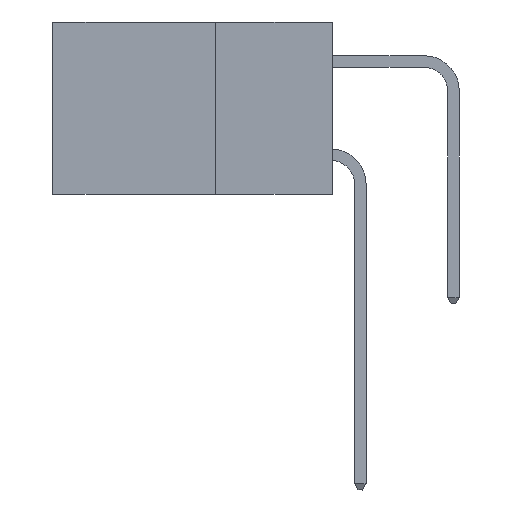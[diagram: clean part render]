
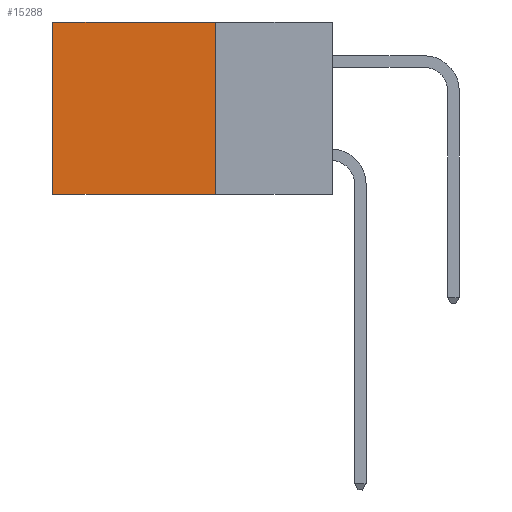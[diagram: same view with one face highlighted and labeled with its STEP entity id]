
A CAD part, left-side view. The second image highlights one B-rep face of the part: STEP entity #15288.
In plain terms, the highlighted planar face has unit normal (-1, 0, 0).
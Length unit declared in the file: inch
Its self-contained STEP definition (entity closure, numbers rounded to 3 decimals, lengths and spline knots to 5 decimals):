
#237 = CARTESIAN_POINT ( 'NONE',  ( 0.2615, 0.6, -0.37 ) ) ;
#735 = VERTEX_POINT ( 'NONE', #8768 ) ;
#882 = EDGE_CURVE ( 'NONE', #735, #15357, #3369, .T. ) ;
#1232 = VECTOR ( 'NONE', #13701, 39.37008 ) ;
#1539 = CARTESIAN_POINT ( 'NONE',  ( 0.2615, 0.6, 0. ) ) ;
#2678 = LINE ( 'NONE', #19272, #17702 ) ;
#2715 = ORIENTED_EDGE ( 'NONE', *, *, #5434, .F. ) ;
#2797 = DIRECTION ( 'NONE',  ( 0., 0., -1. ) ) ;
#2817 = LINE ( 'NONE', #7507, #16532 ) ;
#3369 = LINE ( 'NONE', #16839, #11816 ) ;
#3774 = EDGE_CURVE ( 'NONE', #735, #16047, #2678, .T. ) ;
#3969 = ORIENTED_EDGE ( 'NONE', *, *, #882, .F. ) ;
#4249 = CARTESIAN_POINT ( 'NONE',  ( 0.2615, 0.25, -0.37 ) ) ;
#5434 = EDGE_CURVE ( 'NONE', #15357, #15599, #2817, .T. ) ;
#5747 = CARTESIAN_POINT ( 'NONE',  ( 0.2615, 0.25, -0.37 ) ) ;
#6977 = DIRECTION ( 'NONE',  ( 0., 1., 0. ) ) ;
#7190 = ORIENTED_EDGE ( 'NONE', *, *, #8934, .T. ) ;
#7507 = CARTESIAN_POINT ( 'NONE',  ( 0.2615, 0.25, -0.37 ) ) ;
#8630 = DIRECTION ( 'NONE',  ( 0., 0., -1. ) ) ;
#8768 = CARTESIAN_POINT ( 'NONE',  ( 0.2615, 0.25, 0. ) ) ;
#8934 = EDGE_CURVE ( 'NONE', #16047, #15599, #16800, .T. ) ;
#9025 = PLANE ( 'NONE',  #16343 ) ;
#11723 = DIRECTION ( 'NONE',  ( 1., 0., 0. ) ) ;
#11816 = VECTOR ( 'NONE', #2797, 39.37008 ) ;
#12536 = CARTESIAN_POINT ( 'NONE',  ( 0.2615, 0.6, -0.37 ) ) ;
#13701 = DIRECTION ( 'NONE',  ( 0., 0., -1. ) ) ;
#15288 = ADVANCED_FACE ( 'NONE', ( #16522 ), #9025, .F. ) ;
#15357 = VERTEX_POINT ( 'NONE', #4249 ) ;
#15599 = VERTEX_POINT ( 'NONE', #12536 ) ;
#16047 = VERTEX_POINT ( 'NONE', #1539 ) ;
#16343 = AXIS2_PLACEMENT_3D ( 'NONE', #5747, #11723, #8630 ) ;
#16389 = DIRECTION ( 'NONE',  ( 0., 1., 0. ) ) ;
#16522 = FACE_OUTER_BOUND ( 'NONE', #17247, .T. ) ;
#16532 = VECTOR ( 'NONE', #16389, 39.37008 ) ;
#16800 = LINE ( 'NONE', #237, #1232 ) ;
#16839 = CARTESIAN_POINT ( 'NONE',  ( 0.2615, 0.25, -0.37 ) ) ;
#17247 = EDGE_LOOP ( 'NONE', ( #7190, #2715, #3969, #18802 ) ) ;
#17702 = VECTOR ( 'NONE', #6977, 39.37008 ) ;
#18802 = ORIENTED_EDGE ( 'NONE', *, *, #3774, .T. ) ;
#19272 = CARTESIAN_POINT ( 'NONE',  ( 0.2615, 0.25, 0. ) ) ;
